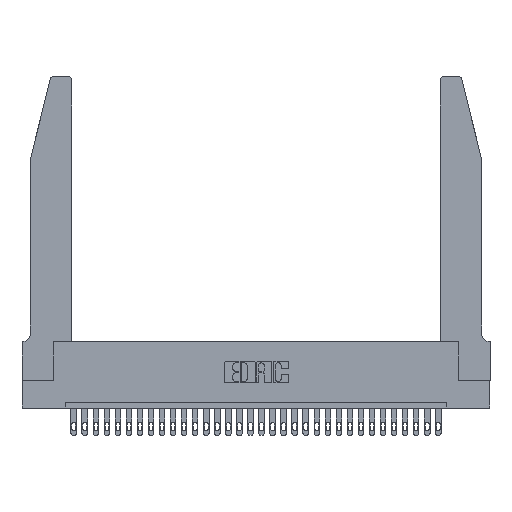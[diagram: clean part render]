
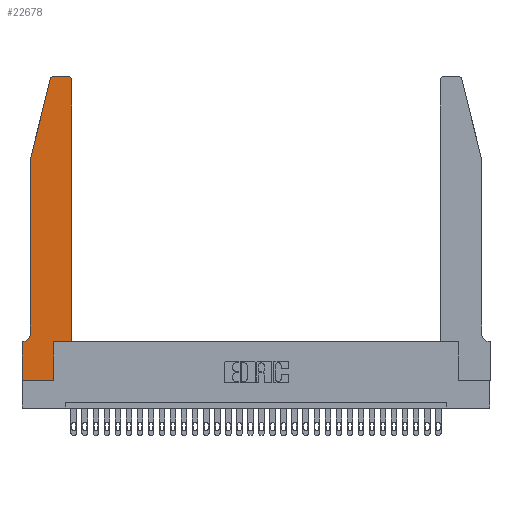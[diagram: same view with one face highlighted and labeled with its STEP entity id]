
A CAD part, top view. The second image highlights one B-rep face of the part: STEP entity #22678.
In plain terms, the highlighted planar face has unit normal (0, 0, 1).
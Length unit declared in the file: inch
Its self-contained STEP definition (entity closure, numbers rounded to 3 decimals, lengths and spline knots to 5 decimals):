
#178 = EDGE_CURVE ( 'NONE', #27016, #19605, #25007, .T. ) ;
#248 = ORIENTED_EDGE ( 'NONE', *, *, #11182, .T. ) ;
#419 = EDGE_CURVE ( 'NONE', #19605, #29854, #21643, .T. ) ;
#568 = VECTOR ( 'NONE', #8761, 39.37008 ) ;
#601 = CARTESIAN_POINT ( 'NONE',  ( 0., 0., 0.37 ) ) ;
#628 = DIRECTION ( 'NONE',  ( 1., 0., 0. ) ) ;
#683 = DIRECTION ( 'NONE',  ( -1., 0., 0. ) ) ;
#1114 = CARTESIAN_POINT ( 'NONE',  ( 0.0055, 0.42, 0.37 ) ) ;
#1500 = CARTESIAN_POINT ( 'NONE',  ( 0.4505, 2.72, 0.37 ) ) ;
#1651 = ORIENTED_EDGE ( 'NONE', *, *, #178, .T. ) ;
#1678 = CARTESIAN_POINT ( 'NONE',  ( 0., 0., 0.37 ) ) ;
#1712 = CARTESIAN_POINT ( 'NONE',  ( 0.0755, 0.35, 0.37 ) ) ;
#2247 = VERTEX_POINT ( 'NONE', #13266 ) ;
#2311 = VECTOR ( 'NONE', #22092, 39.37008 ) ;
#3130 = ORIENTED_EDGE ( 'NONE', *, *, #21613, .T. ) ;
#3391 = ORIENTED_EDGE ( 'NONE', *, *, #19727, .T. ) ;
#3393 = DIRECTION ( 'NONE',  ( 0., 0., 1. ) ) ;
#3765 = AXIS2_PLACEMENT_3D ( 'NONE', #1114, #27546, #683 ) ;
#3783 = CARTESIAN_POINT ( 'NONE',  ( 0.284, 2.75, 0.37 ) ) ;
#4451 = CARTESIAN_POINT ( 'NONE',  ( 0.0755, 2., 0.37 ) ) ;
#4602 = VERTEX_POINT ( 'NONE', #30289 ) ;
#5454 = DIRECTION ( 'NONE',  ( 0., 0., 1. ) ) ;
#5895 = ORIENTED_EDGE ( 'NONE', *, *, #419, .T. ) ;
#6796 = DIRECTION ( 'NONE',  ( -1., 0., 0. ) ) ;
#7177 = ORIENTED_EDGE ( 'NONE', *, *, #20508, .T. ) ;
#7393 = LINE ( 'NONE', #4451, #25993 ) ;
#8761 = DIRECTION ( 'NONE',  ( 1., 0., 0. ) ) ;
#9257 = EDGE_LOOP ( 'NONE', ( #3391, #248, #30845, #14592, #14720, #7177, #1651, #5895, #23548, #25086, #3130, #30591 ) ) ;
#9351 = PLANE ( 'NONE',  #16403 ) ;
#9699 = AXIS2_PLACEMENT_3D ( 'NONE', #22428, #3393, #628 ) ;
#10051 = DIRECTION ( 'NONE',  ( -0.239, -0.971, 0. ) ) ;
#10377 = EDGE_CURVE ( 'NONE', #30368, #2247, #7393, .T. ) ;
#10404 = VECTOR ( 'NONE', #6796, 39.37008 ) ;
#10817 = LINE ( 'NONE', #1712, #10404 ) ;
#11182 = EDGE_CURVE ( 'NONE', #24417, #12613, #17294, .T. ) ;
#11757 = LINE ( 'NONE', #24759, #30655 ) ;
#11811 = DIRECTION ( 'NONE',  ( 1., 0., 0. ) ) ;
#12447 = LINE ( 'NONE', #18239, #20815 ) ;
#12613 = VERTEX_POINT ( 'NONE', #26203 ) ;
#13055 = CARTESIAN_POINT ( 'NONE',  ( 0.2605, 2.75, 0.37 ) ) ;
#13266 = CARTESIAN_POINT ( 'NONE',  ( 0.0755, 0.42, 0.37 ) ) ;
#13383 = DIRECTION ( 'NONE',  ( 0., 1., 0. ) ) ;
#13576 = LINE ( 'NONE', #27874, #25695 ) ;
#14205 = AXIS2_PLACEMENT_3D ( 'NONE', #17662, #5454, #20088 ) ;
#14410 = CARTESIAN_POINT ( 'NONE',  ( 0., 0.35, 0.37 ) ) ;
#14592 = ORIENTED_EDGE ( 'NONE', *, *, #10377, .T. ) ;
#14614 = CARTESIAN_POINT ( 'NONE',  ( 0.2865, 0., 0.37 ) ) ;
#14720 = ORIENTED_EDGE ( 'NONE', *, *, #30943, .T. ) ;
#14769 = CARTESIAN_POINT ( 'NONE',  ( 0., 0., 0.37 ) ) ;
#14800 = CIRCLE ( 'NONE', #3765, 0.07 ) ;
#14900 = EDGE_CURVE ( 'NONE', #29854, #4602, #12447, .T. ) ;
#14907 = CARTESIAN_POINT ( 'NONE',  ( 0.0055, 0.35, 0.37 ) ) ;
#14933 = CARTESIAN_POINT ( 'NONE',  ( 0.4205, 2.75, 0.37 ) ) ;
#15396 = VECTOR ( 'NONE', #15402, 39.37008 ) ;
#15402 = DIRECTION ( 'NONE',  ( -1., 0., 0. ) ) ;
#16403 = AXIS2_PLACEMENT_3D ( 'NONE', #28331, #30952, #11811 ) ;
#17294 = CIRCLE ( 'NONE', #9699, 0.03 ) ;
#17662 = CARTESIAN_POINT ( 'NONE',  ( 0.4205, 2.72, 0.37 ) ) ;
#17787 = EDGE_CURVE ( 'NONE', #12613, #30368, #11757, .T. ) ;
#17862 = VERTEX_POINT ( 'NONE', #14933 ) ;
#18239 = CARTESIAN_POINT ( 'NONE',  ( 0.2865, 0.35, 0.37 ) ) ;
#18451 = CARTESIAN_POINT ( 'NONE',  ( 0.0755, 2., 0.37 ) ) ;
#18972 = CARTESIAN_POINT ( 'NONE',  ( 0.4505, 0.35, 0.37 ) ) ;
#19304 = FACE_OUTER_BOUND ( 'NONE', #9257, .T. ) ;
#19605 = VERTEX_POINT ( 'NONE', #14769 ) ;
#19727 = EDGE_CURVE ( 'NONE', #17862, #24417, #30144, .T. ) ;
#20088 = DIRECTION ( 'NONE',  ( 1., 0., 0. ) ) ;
#20508 = EDGE_CURVE ( 'NONE', #20818, #27016, #10817, .T. ) ;
#20815 = VECTOR ( 'NONE', #27919, 39.37008 ) ;
#20818 = VERTEX_POINT ( 'NONE', #14907 ) ;
#21191 = VERTEX_POINT ( 'NONE', #18972 ) ;
#21488 = DIRECTION ( 'NONE',  ( 0., -1., 0. ) ) ;
#21613 = EDGE_CURVE ( 'NONE', #21191, #23241, #13576, .T. ) ;
#21643 = LINE ( 'NONE', #601, #2311 ) ;
#22092 = DIRECTION ( 'NONE',  ( 1., 0., 0. ) ) ;
#22428 = CARTESIAN_POINT ( 'NONE',  ( 0.284, 2.72, 0.37 ) ) ;
#22678 = ADVANCED_FACE ( 'NONE', ( #19304 ), #9351, .T. ) ;
#23241 = VERTEX_POINT ( 'NONE', #1500 ) ;
#23548 = ORIENTED_EDGE ( 'NONE', *, *, #14900, .T. ) ;
#23945 = EDGE_CURVE ( 'NONE', #4602, #21191, #31254, .T. ) ;
#24372 = EDGE_CURVE ( 'NONE', #23241, #17862, #28614, .T. ) ;
#24417 = VERTEX_POINT ( 'NONE', #3783 ) ;
#24759 = CARTESIAN_POINT ( 'NONE',  ( 0.0755, 2., 0.37 ) ) ;
#25007 = LINE ( 'NONE', #1678, #26877 ) ;
#25086 = ORIENTED_EDGE ( 'NONE', *, *, #23945, .T. ) ;
#25607 = CARTESIAN_POINT ( 'NONE',  ( 0.4505, 0.35, 0.37 ) ) ;
#25695 = VECTOR ( 'NONE', #13383, 39.37008 ) ;
#25993 = VECTOR ( 'NONE', #26013, 39.37008 ) ;
#26013 = DIRECTION ( 'NONE',  ( 0., -1., 0. ) ) ;
#26203 = CARTESIAN_POINT ( 'NONE',  ( 0.25487, 2.72718, 0.37 ) ) ;
#26877 = VECTOR ( 'NONE', #21488, 39.37008 ) ;
#27016 = VERTEX_POINT ( 'NONE', #14410 ) ;
#27546 = DIRECTION ( 'NONE',  ( 0., 0., -1. ) ) ;
#27874 = CARTESIAN_POINT ( 'NONE',  ( 0.4505, 0.35, 0.37 ) ) ;
#27919 = DIRECTION ( 'NONE',  ( 0., 1., 0. ) ) ;
#28331 = CARTESIAN_POINT ( 'NONE',  ( 0., 0.35, 0.37 ) ) ;
#28614 = CIRCLE ( 'NONE', #14205, 0.03 ) ;
#29854 = VERTEX_POINT ( 'NONE', #14614 ) ;
#30144 = LINE ( 'NONE', #13055, #15396 ) ;
#30289 = CARTESIAN_POINT ( 'NONE',  ( 0.2865, 0.35, 0.37 ) ) ;
#30368 = VERTEX_POINT ( 'NONE', #18451 ) ;
#30591 = ORIENTED_EDGE ( 'NONE', *, *, #24372, .T. ) ;
#30655 = VECTOR ( 'NONE', #10051, 39.37008 ) ;
#30845 = ORIENTED_EDGE ( 'NONE', *, *, #17787, .T. ) ;
#30943 = EDGE_CURVE ( 'NONE', #2247, #20818, #14800, .T. ) ;
#30952 = DIRECTION ( 'NONE',  ( 0., 0., 1. ) ) ;
#31254 = LINE ( 'NONE', #25607, #568 ) ;
